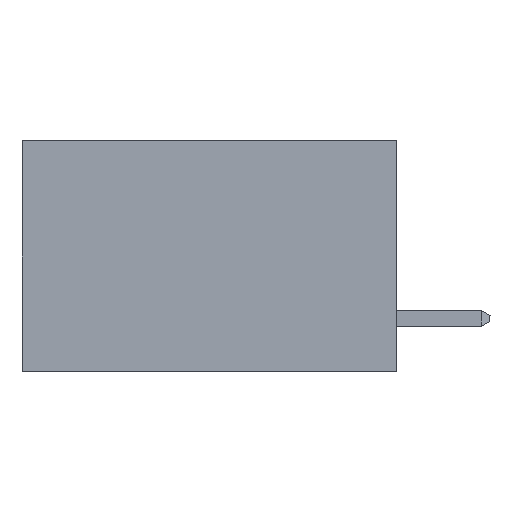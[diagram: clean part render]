
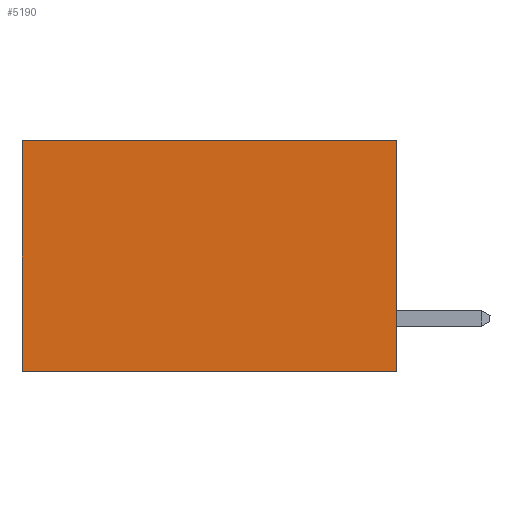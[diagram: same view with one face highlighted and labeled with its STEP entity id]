
A CAD part, left-side view. The second image highlights one B-rep face of the part: STEP entity #5190.
In plain terms, the highlighted planar face has unit normal (-1, 0, 0).
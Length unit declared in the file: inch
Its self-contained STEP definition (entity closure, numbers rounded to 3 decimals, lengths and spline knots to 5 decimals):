
#137 = CARTESIAN_POINT ( 'NONE',  ( 0.2615, 0., 0. ) ) ;
#371 = EDGE_CURVE ( 'NONE', #2192, #1895, #3835, .T. ) ;
#694 = DIRECTION ( 'NONE',  ( 0., 1., 0. ) ) ;
#1542 = CARTESIAN_POINT ( 'NONE',  ( 0.2615, 0.6, 0. ) ) ;
#1565 = CARTESIAN_POINT ( 'NONE',  ( 0.2615, 0.6, -0.37 ) ) ;
#1895 = VERTEX_POINT ( 'NONE', #8236 ) ;
#2192 = VERTEX_POINT ( 'NONE', #8715 ) ;
#2293 = PLANE ( 'NONE',  #8405 ) ;
#2334 = DIRECTION ( 'NONE',  ( 0., 1., 0. ) ) ;
#2336 = DIRECTION ( 'NONE',  ( 1., 0., 0. ) ) ;
#2344 = LINE ( 'NONE', #7950, #4731 ) ;
#2472 = FACE_OUTER_BOUND ( 'NONE', #8294, .T. ) ;
#2510 = VECTOR ( 'NONE', #2334, 39.37008 ) ;
#3108 = VERTEX_POINT ( 'NONE', #1565 ) ;
#3649 = VECTOR ( 'NONE', #4659, 39.37008 ) ;
#3835 = LINE ( 'NONE', #6768, #3649 ) ;
#4659 = DIRECTION ( 'NONE',  ( 0., 0., -1. ) ) ;
#4690 = EDGE_CURVE ( 'NONE', #7520, #3108, #2344, .T. ) ;
#4731 = VECTOR ( 'NONE', #8654, 39.37008 ) ;
#5092 = CARTESIAN_POINT ( 'NONE',  ( 0.2615, 0., -0.37 ) ) ;
#5134 = DIRECTION ( 'NONE',  ( 0., 0., -1. ) ) ;
#5190 = ADVANCED_FACE ( 'NONE', ( #2472 ), #2293, .F. ) ;
#6240 = VECTOR ( 'NONE', #694, 39.37008 ) ;
#6287 = EDGE_CURVE ( 'NONE', #1895, #3108, #6999, .T. ) ;
#6556 = LINE ( 'NONE', #137, #2510 ) ;
#6768 = CARTESIAN_POINT ( 'NONE',  ( 0.2615, 0., -0.37 ) ) ;
#6914 = ORIENTED_EDGE ( 'NONE', *, *, #6287, .F. ) ;
#6945 = ORIENTED_EDGE ( 'NONE', *, *, #371, .F. ) ;
#6999 = LINE ( 'NONE', #8318, #6240 ) ;
#7520 = VERTEX_POINT ( 'NONE', #1542 ) ;
#7950 = CARTESIAN_POINT ( 'NONE',  ( 0.2615, 0.6, -0.37 ) ) ;
#8214 = ORIENTED_EDGE ( 'NONE', *, *, #8839, .T. ) ;
#8236 = CARTESIAN_POINT ( 'NONE',  ( 0.2615, 0., -0.37 ) ) ;
#8294 = EDGE_LOOP ( 'NONE', ( #8473, #6914, #6945, #8214 ) ) ;
#8318 = CARTESIAN_POINT ( 'NONE',  ( 0.2615, 0., -0.37 ) ) ;
#8405 = AXIS2_PLACEMENT_3D ( 'NONE', #5092, #2336, #5134 ) ;
#8473 = ORIENTED_EDGE ( 'NONE', *, *, #4690, .T. ) ;
#8654 = DIRECTION ( 'NONE',  ( 0., 0., -1. ) ) ;
#8715 = CARTESIAN_POINT ( 'NONE',  ( 0.2615, 0., 0. ) ) ;
#8839 = EDGE_CURVE ( 'NONE', #2192, #7520, #6556, .T. ) ;
